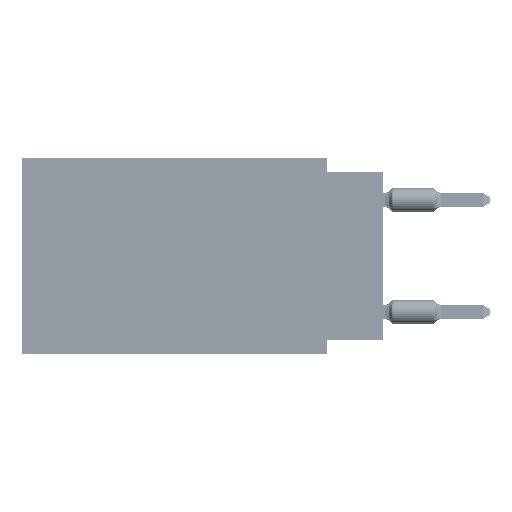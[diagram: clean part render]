
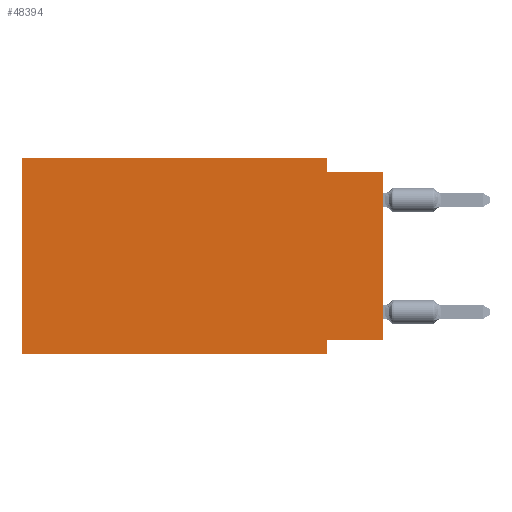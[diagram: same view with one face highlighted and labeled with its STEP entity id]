
A CAD part, left-side view. The second image highlights one B-rep face of the part: STEP entity #48394.
In plain terms, the highlighted planar face has unit normal (-1, 0, 0).
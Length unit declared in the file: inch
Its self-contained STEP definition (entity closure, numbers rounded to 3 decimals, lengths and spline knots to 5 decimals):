
#209 = CARTESIAN_POINT ( 'NONE',  ( 0., 0.645, 0. ) ) ;
#413 = CARTESIAN_POINT ( 'NONE',  ( 0., 0., -0.025 ) ) ;
#2463 = VECTOR ( 'NONE', #49590, 39.37008 ) ;
#4753 = DIRECTION ( 'NONE',  ( 0., -1., 0. ) ) ;
#5349 = VERTEX_POINT ( 'NONE', #48132 ) ;
#5484 = LINE ( 'NONE', #209, #56704 ) ;
#7648 = VECTOR ( 'NONE', #57270, 39.37008 ) ;
#8501 = LINE ( 'NONE', #25277, #36741 ) ;
#8856 = DIRECTION ( 'NONE',  ( 0., 0., -1. ) ) ;
#8937 = CARTESIAN_POINT ( 'NONE',  ( 0., 0., -0.325 ) ) ;
#12153 = CARTESIAN_POINT ( 'NONE',  ( 0., 0.1, -0.325 ) ) ;
#16222 = VECTOR ( 'NONE', #31625, 39.37008 ) ;
#16304 = DIRECTION ( 'NONE',  ( 0., 0., -1. ) ) ;
#16981 = PLANE ( 'NONE',  #44156 ) ;
#18056 = EDGE_CURVE ( 'NONE', #63150, #68614, #8501, .T. ) ;
#18700 = VERTEX_POINT ( 'NONE', #58505 ) ;
#18942 = CARTESIAN_POINT ( 'NONE',  ( 0., 0.1, -0.35 ) ) ;
#20162 = LINE ( 'NONE', #68499, #35178 ) ;
#20249 = EDGE_LOOP ( 'NONE', ( #46114, #56016, #60216, #41010, #43042, #65183, #30276, #36368 ) ) ;
#21495 = EDGE_CURVE ( 'NONE', #18700, #63150, #67772, .T. ) ;
#21525 = DIRECTION ( 'NONE',  ( 0., -1., 0. ) ) ;
#25277 = CARTESIAN_POINT ( 'NONE',  ( 0., 0.1, -0.35 ) ) ;
#25333 = CARTESIAN_POINT ( 'NONE',  ( 0., 0.1, 0. ) ) ;
#28519 = CARTESIAN_POINT ( 'NONE',  ( 0., 0.1, 0. ) ) ;
#28735 = CARTESIAN_POINT ( 'NONE',  ( 0., 0.645, 0. ) ) ;
#29069 = VERTEX_POINT ( 'NONE', #54990 ) ;
#30276 = ORIENTED_EDGE ( 'NONE', *, *, #18056, .F. ) ;
#31625 = DIRECTION ( 'NONE',  ( 0., 0., -1. ) ) ;
#33493 = LINE ( 'NONE', #48247, #2463 ) ;
#35011 = LINE ( 'NONE', #28735, #57642 ) ;
#35178 = VECTOR ( 'NONE', #4753, 39.37008 ) ;
#35384 = VECTOR ( 'NONE', #52640, 39.37008 ) ;
#36368 = ORIENTED_EDGE ( 'NONE', *, *, #21495, .F. ) ;
#36741 = VECTOR ( 'NONE', #8856, 39.37008 ) ;
#38525 = EDGE_CURVE ( 'NONE', #29069, #51573, #35011, .T. ) ;
#40559 = VERTEX_POINT ( 'NONE', #413 ) ;
#41010 = ORIENTED_EDGE ( 'NONE', *, *, #65909, .F. ) ;
#42871 = EDGE_CURVE ( 'NONE', #18700, #40559, #48395, .T. ) ;
#43042 = ORIENTED_EDGE ( 'NONE', *, *, #38525, .F. ) ;
#44156 = AXIS2_PLACEMENT_3D ( 'NONE', #53450, #53086, #16304 ) ;
#46114 = ORIENTED_EDGE ( 'NONE', *, *, #42871, .T. ) ;
#48132 = CARTESIAN_POINT ( 'NONE',  ( 0., 0.1, -0.025 ) ) ;
#48247 = CARTESIAN_POINT ( 'NONE',  ( 0., 0., -0.025 ) ) ;
#48394 = ADVANCED_FACE ( 'NONE', ( #64639 ), #16981, .F. ) ;
#48395 = LINE ( 'NONE', #53337, #35384 ) ;
#49590 = DIRECTION ( 'NONE',  ( 0., -1., 0. ) ) ;
#51156 = DIRECTION ( 'NONE',  ( 0., 0., 1. ) ) ;
#51573 = VERTEX_POINT ( 'NONE', #57491 ) ;
#52640 = DIRECTION ( 'NONE',  ( 0., 0., 1. ) ) ;
#53086 = DIRECTION ( 'NONE',  ( 1., 0., 0. ) ) ;
#53337 = CARTESIAN_POINT ( 'NONE',  ( 0., 0., 0. ) ) ;
#53450 = CARTESIAN_POINT ( 'NONE',  ( 0., 0.645, 0. ) ) ;
#54157 = EDGE_CURVE ( 'NONE', #5349, #40559, #33493, .T. ) ;
#54990 = CARTESIAN_POINT ( 'NONE',  ( 0., 0.645, -0.35 ) ) ;
#56016 = ORIENTED_EDGE ( 'NONE', *, *, #54157, .F. ) ;
#56704 = VECTOR ( 'NONE', #21525, 39.37008 ) ;
#57270 = DIRECTION ( 'NONE',  ( 0., 1., 0. ) ) ;
#57491 = CARTESIAN_POINT ( 'NONE',  ( 0., 0.645, 0. ) ) ;
#57642 = VECTOR ( 'NONE', #51156, 39.37008 ) ;
#58505 = CARTESIAN_POINT ( 'NONE',  ( 0., 0., -0.325 ) ) ;
#59472 = EDGE_CURVE ( 'NONE', #66073, #5349, #63539, .T. ) ;
#60216 = ORIENTED_EDGE ( 'NONE', *, *, #59472, .F. ) ;
#63150 = VERTEX_POINT ( 'NONE', #12153 ) ;
#63459 = EDGE_CURVE ( 'NONE', #29069, #68614, #20162, .T. ) ;
#63539 = LINE ( 'NONE', #25333, #16222 ) ;
#64639 = FACE_OUTER_BOUND ( 'NONE', #20249, .T. ) ;
#65183 = ORIENTED_EDGE ( 'NONE', *, *, #63459, .T. ) ;
#65909 = EDGE_CURVE ( 'NONE', #51573, #66073, #5484, .T. ) ;
#66073 = VERTEX_POINT ( 'NONE', #28519 ) ;
#67772 = LINE ( 'NONE', #8937, #7648 ) ;
#68499 = CARTESIAN_POINT ( 'NONE',  ( 0., 0.645, -0.35 ) ) ;
#68614 = VERTEX_POINT ( 'NONE', #18942 ) ;
